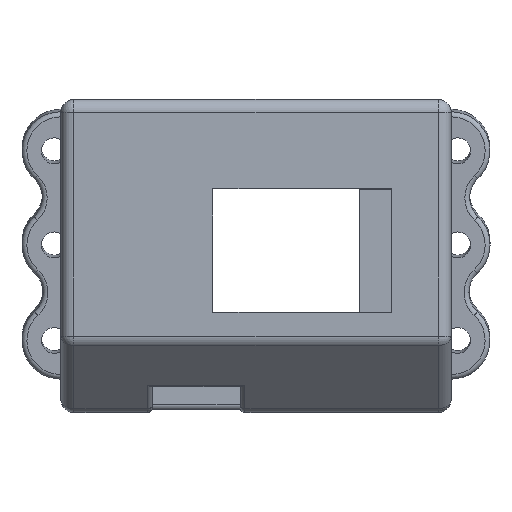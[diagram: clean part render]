
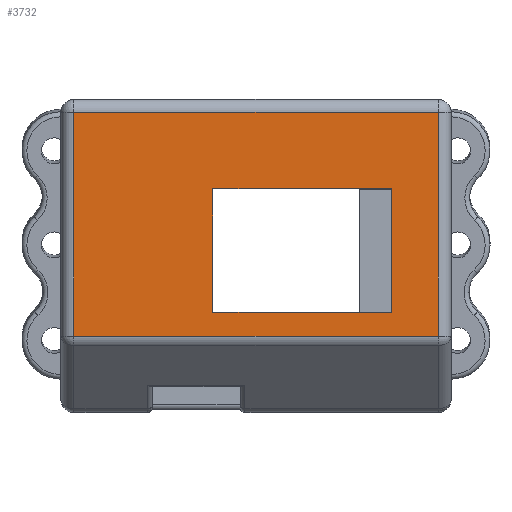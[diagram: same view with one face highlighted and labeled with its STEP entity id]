
A CAD part, top view. The second image highlights one B-rep face of the part: STEP entity #3732.
In plain terms, the highlighted planar face has unit normal (0, 0, 1).
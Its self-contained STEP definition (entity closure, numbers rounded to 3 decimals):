
#134=FACE_BOUND('',#802,.T.);
#573=FACE_OUTER_BOUND('',#801,.T.);
#801=EDGE_LOOP('',(#2656,#2657,#2658,#2659));
#802=EDGE_LOOP('',(#2660,#2661,#2662,#2663));
#1116=LINE('',#5839,#1364);
#1148=LINE('',#5909,#1396);
#1150=LINE('',#5914,#1398);
#1151=LINE('',#5916,#1399);
#1152=LINE('',#5918,#1400);
#1153=LINE('',#5919,#1401);
#1154=LINE('',#5920,#1402);
#1155=LINE('',#5921,#1403);
#1364=VECTOR('',#4571,10.);
#1396=VECTOR('',#4627,10.);
#1398=VECTOR('',#4631,10.);
#1399=VECTOR('',#4632,10.);
#1400=VECTOR('',#4633,10.);
#1401=VECTOR('',#4634,10.);
#1402=VECTOR('',#4635,10.);
#1403=VECTOR('',#4636,10.);
#1621=VERTEX_POINT('',#5836);
#1622=VERTEX_POINT('',#5838);
#1647=VERTEX_POINT('',#5906);
#1648=VERTEX_POINT('',#5908);
#1649=VERTEX_POINT('',#5912);
#1650=VERTEX_POINT('',#5913);
#1651=VERTEX_POINT('',#5915);
#1652=VERTEX_POINT('',#5917);
#2000=EDGE_CURVE('',#1622,#1621,#1116,.T.);
#2036=EDGE_CURVE('',#1648,#1647,#1148,.T.);
#2038=EDGE_CURVE('',#1649,#1650,#1150,.T.);
#2039=EDGE_CURVE('',#1651,#1649,#1151,.T.);
#2040=EDGE_CURVE('',#1652,#1651,#1152,.T.);
#2041=EDGE_CURVE('',#1650,#1652,#1153,.T.);
#2042=EDGE_CURVE('',#1621,#1648,#1154,.T.);
#2043=EDGE_CURVE('',#1647,#1622,#1155,.T.);
#2656=ORIENTED_EDGE('',*,*,#2038,.F.);
#2657=ORIENTED_EDGE('',*,*,#2039,.F.);
#2658=ORIENTED_EDGE('',*,*,#2040,.F.);
#2659=ORIENTED_EDGE('',*,*,#2041,.F.);
#2660=ORIENTED_EDGE('',*,*,#2042,.T.);
#2661=ORIENTED_EDGE('',*,*,#2036,.T.);
#2662=ORIENTED_EDGE('',*,*,#2043,.T.);
#2663=ORIENTED_EDGE('',*,*,#2000,.T.);
#3659=PLANE('',#3999);
#3732=ADVANCED_FACE('',(#573,#134),#3659,.T.);
#3999=AXIS2_PLACEMENT_3D('',#5911,#4629,#4630);
#4571=DIRECTION('',(1.,0.,0.));
#4627=DIRECTION('',(-1.,0.,0.));
#4629=DIRECTION('center_axis',(0.,0.,1.));
#4630=DIRECTION('ref_axis',(1.,0.,0.));
#4631=DIRECTION('',(-1.,0.,0.));
#4632=DIRECTION('',(0.,-1.,0.));
#4633=DIRECTION('',(1.,0.,0.));
#4634=DIRECTION('',(0.,1.,0.));
#4635=DIRECTION('',(0.,-1.,0.));
#4636=DIRECTION('',(0.,1.,0.));
#5836=CARTESIAN_POINT('',(20.956,-13.887,267.));
#5838=CARTESIAN_POINT('',(-6.656,-13.887,267.));
#5839=CARTESIAN_POINT('',(-6.656,-13.887,267.));
#5906=CARTESIAN_POINT('',(-6.656,-32.934,267.));
#5908=CARTESIAN_POINT('',(20.956,-32.934,267.));
#5909=CARTESIAN_POINT('',(10.478,-32.934,267.));
#5911=CARTESIAN_POINT('Origin',(0.,-24.313,267.));
#5912=CARTESIAN_POINT('',(28.1,-36.614,267.));
#5913=CARTESIAN_POINT('',(-28.1,-36.614,267.));
#5914=CARTESIAN_POINT('',(5.8,-36.614,267.));
#5915=CARTESIAN_POINT('',(28.1,-2.086,267.));
#5916=CARTESIAN_POINT('',(28.1,-24.313,267.));
#5917=CARTESIAN_POINT('',(-28.1,-2.086,267.));
#5918=CARTESIAN_POINT('',(8.05,-2.086,267.));
#5919=CARTESIAN_POINT('',(-28.1,-24.313,267.));
#5920=CARTESIAN_POINT('',(20.956,-0.086,267.));
#5921=CARTESIAN_POINT('',(-6.656,-32.055,267.));
